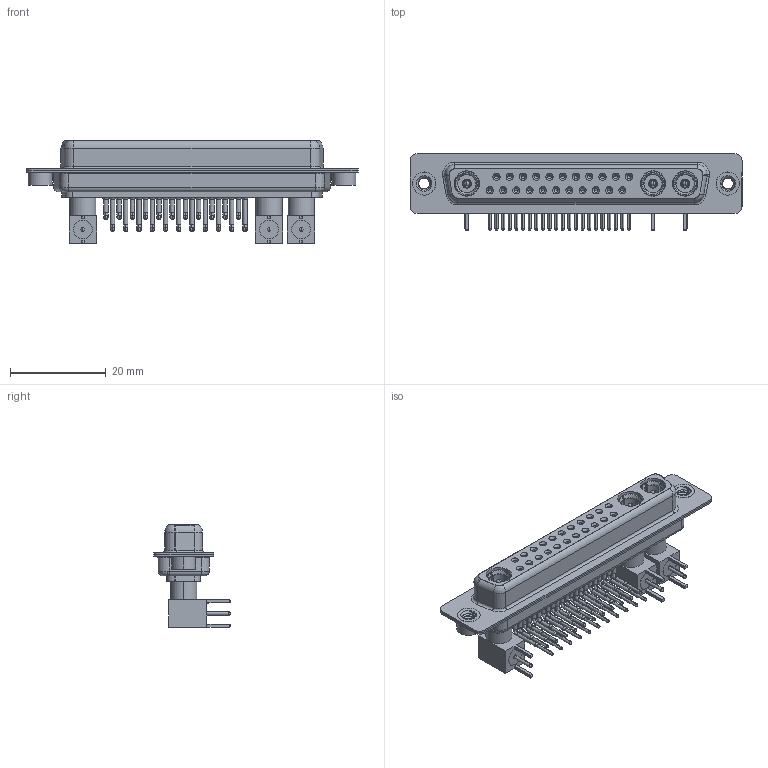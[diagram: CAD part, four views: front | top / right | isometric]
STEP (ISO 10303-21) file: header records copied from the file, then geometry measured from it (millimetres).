
FILE_DESCRIPTION (( 'STEP AP203' ), '1' );
FILE_NAME ('630-25W3640-5T2.STEP', '2022-06-07T08:19:24', ( '' ), ( '' ), 'SwSTEP 2.0', 'SolidWorks 2020', '' );
FILE_SCHEMA (( 'CONFIG_CONTROL_DESIGN' ));
Length unit declared in the file: millimetre
Products named in the file (16): Locking Collar; 630Combo Shell Front_37 Contacts; Insulator RA Pin; 630Combo Housing_25W3; 630Combo Threaded Rivet_2; Co-Ax Plug Assy_RA; Insulator Pin_Straight PC Tail; RA Back Shell; 630Combo Contact Row 1; Pin_RA; 630-25W3640-5T2; Co-Ax Plug_RA PC Tail; 630Combo Shell Rear_37 Contacts; 630Combo Contact Row 2
Assembly tree (48 placements, depth 3):
  630-25W3640-5T2
    630Combo Housing_25W3
    630Combo Shell Front_37 Contacts
    630Combo Shell Rear_37 Contacts
    630Combo Threaded Rivet_2  x2
    Co-Ax Plug Assy_RA
      Co-Ax Plug_RA PC Tail
      Insulator Pin_Straight PC Tail
      Pin_RA
      Locking Collar
      RA Back Shell
      Insulator RA Pin
    Co-Ax Plug Assy_RA
      Co-Ax Plug_RA PC Tail
      Insulator Pin_Straight PC Tail
      Pin_RA
      Locking Collar
      RA Back Shell
      Insulator RA Pin
    Co-Ax Plug Assy_RA
      Co-Ax Plug_RA PC Tail
      Insulator Pin_Straight PC Tail
      Pin_RA
      Locking Collar
      RA Back Shell
      Insulator RA Pin
    630Combo Contact Row 1  x11
    630Combo Contact Row 2  x11
Bounding box: 69.4 x 16 x 21.41 mm (x, y, z)
Volume: 6173.9 mm3; surface area: 14580.3 mm2
Topology: 45 solids, 45 shells, 1949 faces, 4858 edges, 3050 vertices
Faces by surface type: cylinder 838, plane 598, cone 329, bspline 97, torus 75, sphere 12
Entity records: 27449 total; most frequent: CARTESIAN_POINT 5921, DIRECTION 4358, ORIENTED_EDGE 3678, EDGE_CURVE 1839, AXIS2_PLACEMENT_3D 1806, VERTEX_POINT 1170, CIRCLE 974, EDGE_LOOP 959
